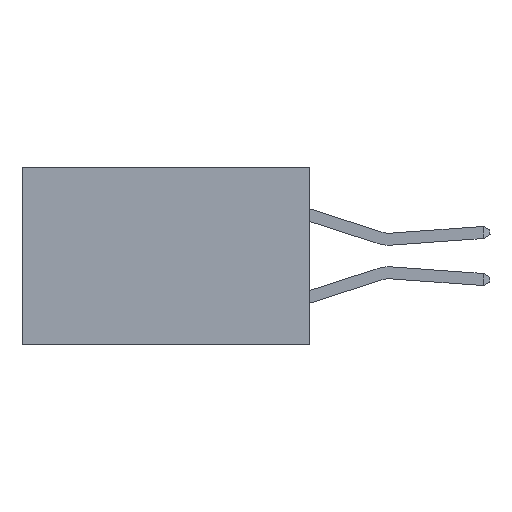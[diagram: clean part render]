
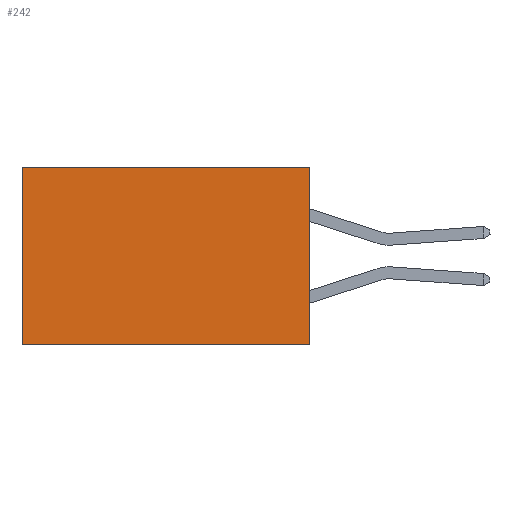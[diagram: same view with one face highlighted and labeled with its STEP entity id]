
A CAD part, left-side view. The second image highlights one B-rep face of the part: STEP entity #242.
In plain terms, the highlighted planar face has unit normal (-1, 0, 0).
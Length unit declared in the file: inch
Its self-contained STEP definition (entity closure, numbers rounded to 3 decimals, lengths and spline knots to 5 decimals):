
#242 = ADVANCED_FACE ( 'NONE', ( #9895 ), #22034, .F. ) ;
#478 = AXIS2_PLACEMENT_3D ( 'NONE', #10111, #20355, #11934 ) ;
#523 = CARTESIAN_POINT ( 'NONE',  ( 0.2615, 0., 0. ) ) ;
#1338 = CARTESIAN_POINT ( 'NONE',  ( 0.2615, 0., 0. ) ) ;
#1678 = DIRECTION ( 'NONE',  ( 0., 0., -1. ) ) ;
#2795 = VERTEX_POINT ( 'NONE', #17361 ) ;
#3603 = VECTOR ( 'NONE', #13639, 39.37008 ) ;
#3917 = EDGE_CURVE ( 'NONE', #22083, #2795, #8105, .T. ) ;
#4857 = LINE ( 'NONE', #1338, #3603 ) ;
#5911 = VECTOR ( 'NONE', #1678, 39.37008 ) ;
#6058 = CARTESIAN_POINT ( 'NONE',  ( 0.2615, 0., -0.37 ) ) ;
#6767 = EDGE_CURVE ( 'NONE', #13149, #15092, #4857, .T. ) ;
#8105 = LINE ( 'NONE', #6058, #18849 ) ;
#8244 = DIRECTION ( 'NONE',  ( 0., 0., -1. ) ) ;
#9208 = CARTESIAN_POINT ( 'NONE',  ( 0.2615, 0., -0.37 ) ) ;
#9895 = FACE_OUTER_BOUND ( 'NONE', #15725, .T. ) ;
#10111 = CARTESIAN_POINT ( 'NONE',  ( 0.2615, 0., -0.37 ) ) ;
#10720 = ORIENTED_EDGE ( 'NONE', *, *, #3917, .F. ) ;
#11597 = EDGE_CURVE ( 'NONE', #15092, #2795, #11710, .T. ) ;
#11710 = LINE ( 'NONE', #20145, #15237 ) ;
#11934 = DIRECTION ( 'NONE',  ( 0., 0., -1. ) ) ;
#13018 = EDGE_CURVE ( 'NONE', #13149, #22083, #19010, .T. ) ;
#13078 = ORIENTED_EDGE ( 'NONE', *, *, #13018, .F. ) ;
#13149 = VERTEX_POINT ( 'NONE', #523 ) ;
#13639 = DIRECTION ( 'NONE',  ( 0., 1., 0. ) ) ;
#15092 = VERTEX_POINT ( 'NONE', #20746 ) ;
#15237 = VECTOR ( 'NONE', #8244, 39.37008 ) ;
#15725 = EDGE_LOOP ( 'NONE', ( #21882, #10720, #13078, #22166 ) ) ;
#17361 = CARTESIAN_POINT ( 'NONE',  ( 0.2615, 0.6, -0.37 ) ) ;
#18418 = DIRECTION ( 'NONE',  ( 0., 1., 0. ) ) ;
#18800 = CARTESIAN_POINT ( 'NONE',  ( 0.2615, 0., -0.37 ) ) ;
#18849 = VECTOR ( 'NONE', #18418, 39.37008 ) ;
#19010 = LINE ( 'NONE', #18800, #5911 ) ;
#20145 = CARTESIAN_POINT ( 'NONE',  ( 0.2615, 0.6, -0.37 ) ) ;
#20355 = DIRECTION ( 'NONE',  ( 1., 0., 0. ) ) ;
#20746 = CARTESIAN_POINT ( 'NONE',  ( 0.2615, 0.6, 0. ) ) ;
#21882 = ORIENTED_EDGE ( 'NONE', *, *, #11597, .T. ) ;
#22034 = PLANE ( 'NONE',  #478 ) ;
#22083 = VERTEX_POINT ( 'NONE', #9208 ) ;
#22166 = ORIENTED_EDGE ( 'NONE', *, *, #6767, .T. ) ;
